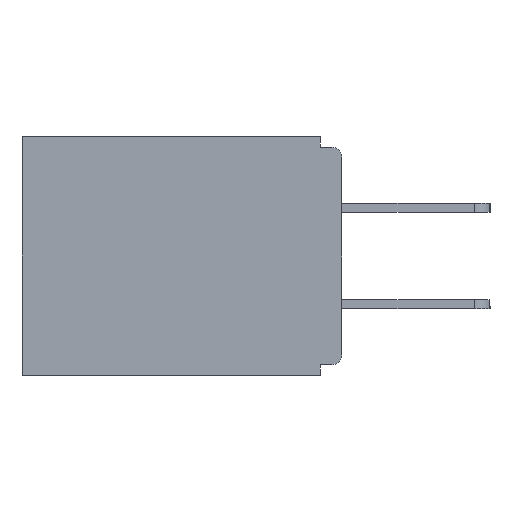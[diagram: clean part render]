
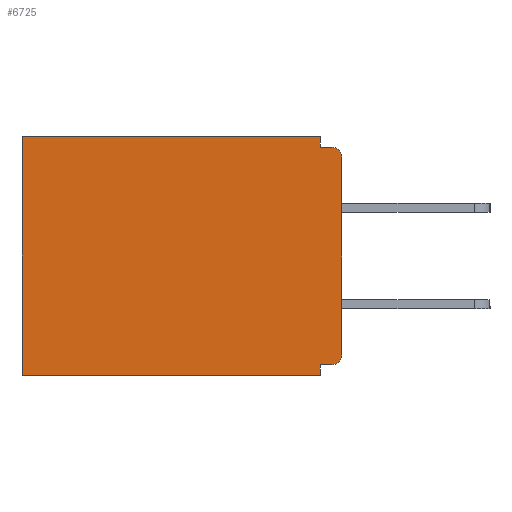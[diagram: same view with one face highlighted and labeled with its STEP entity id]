
A CAD part, left-side view. The second image highlights one B-rep face of the part: STEP entity #6725.
In plain terms, the highlighted planar face has unit normal (-1, 0, 0).
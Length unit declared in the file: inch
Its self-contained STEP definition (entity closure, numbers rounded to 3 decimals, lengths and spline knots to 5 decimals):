
#61 = CARTESIAN_POINT ( 'NONE',  ( 0.298, 0.015, -0.328 ) ) ;
#503 = VERTEX_POINT ( 'NONE', #61 ) ;
#517 = DIRECTION ( 'NONE',  ( 0., 1., 0. ) ) ;
#707 = VECTOR ( 'NONE', #517, 39.37008 ) ;
#1121 = DIRECTION ( 'NONE',  ( -1., 0., 0. ) ) ;
#1235 = AXIS2_PLACEMENT_3D ( 'NONE', #15444, #15633, #13541 ) ;
#2090 = VERTEX_POINT ( 'NONE', #24667 ) ;
#2184 = EDGE_CURVE ( 'NONE', #11422, #6461, #11250, .T. ) ;
#2743 = ORIENTED_EDGE ( 'NONE', *, *, #18848, .F. ) ;
#3019 = ORIENTED_EDGE ( 'NONE', *, *, #14815, .F. ) ;
#3341 = EDGE_CURVE ( 'NONE', #503, #3554, #10534, .T. ) ;
#3554 = VERTEX_POINT ( 'NONE', #15987 ) ;
#3602 = CARTESIAN_POINT ( 'NONE',  ( 0.298, 0.031, -0.343 ) ) ;
#3847 = ORIENTED_EDGE ( 'NONE', *, *, #4492, .F. ) ;
#4006 = CARTESIAN_POINT ( 'NONE',  ( 0.298, 0.015, -0.015 ) ) ;
#4492 = EDGE_CURVE ( 'NONE', #11422, #3554, #22615, .T. ) ;
#4788 = CARTESIAN_POINT ( 'NONE',  ( 0.298, 0., 0. ) ) ;
#5013 = VECTOR ( 'NONE', #8627, 39.37008 ) ;
#5342 = FACE_OUTER_BOUND ( 'NONE', #15247, .T. ) ;
#5429 = DIRECTION ( 'NONE',  ( 0., 1., 0. ) ) ;
#5515 = VERTEX_POINT ( 'NONE', #15365 ) ;
#5703 = EDGE_CURVE ( 'NONE', #17029, #7358, #20069, .T. ) ;
#5813 = ORIENTED_EDGE ( 'NONE', *, *, #6820, .F. ) ;
#6461 = VERTEX_POINT ( 'NONE', #4006 ) ;
#6725 = ADVANCED_FACE ( 'NONE', ( #5342 ), #16725, .F. ) ;
#6820 = EDGE_CURVE ( 'NONE', #2090, #6461, #24026, .T. ) ;
#7358 = VERTEX_POINT ( 'NONE', #18731 ) ;
#7524 = DIRECTION ( 'NONE',  ( 0., 0., -1. ) ) ;
#8010 = AXIS2_PLACEMENT_3D ( 'NONE', #4788, #8545, #16563 ) ;
#8173 = LINE ( 'NONE', #16007, #15008 ) ;
#8213 = ORIENTED_EDGE ( 'NONE', *, *, #20113, .T. ) ;
#8456 = ORIENTED_EDGE ( 'NONE', *, *, #21881, .F. ) ;
#8540 = ORIENTED_EDGE ( 'NONE', *, *, #2184, .T. ) ;
#8545 = DIRECTION ( 'NONE',  ( 1., 0., 0. ) ) ;
#8627 = DIRECTION ( 'NONE',  ( 0., -1., 0. ) ) ;
#8683 = EDGE_CURVE ( 'NONE', #503, #9806, #25272, .T. ) ;
#9072 = DIRECTION ( 'NONE',  ( 0., 0., -1. ) ) ;
#9448 = DIRECTION ( 'NONE',  ( 0., 0., -1. ) ) ;
#9806 = VERTEX_POINT ( 'NONE', #22712 ) ;
#9815 = ORIENTED_EDGE ( 'NONE', *, *, #5703, .T. ) ;
#10089 = DIRECTION ( 'NONE',  ( 0., 0., -1. ) ) ;
#10125 = VECTOR ( 'NONE', #5429, 39.37008 ) ;
#10534 = CIRCLE ( 'NONE', #1235, 0.015 ) ;
#11250 = CIRCLE ( 'NONE', #18789, 0.015 ) ;
#11393 = CARTESIAN_POINT ( 'NONE',  ( 0.298, 0., -0.343 ) ) ;
#11422 = VERTEX_POINT ( 'NONE', #11883 ) ;
#11802 = VECTOR ( 'NONE', #7524, 39.37008 ) ;
#11831 = CARTESIAN_POINT ( 'NONE',  ( 0.298, 0.46, 0. ) ) ;
#11869 = ORIENTED_EDGE ( 'NONE', *, *, #3341, .T. ) ;
#11883 = CARTESIAN_POINT ( 'NONE',  ( 0.298, 0., -0.03 ) ) ;
#13541 = DIRECTION ( 'NONE',  ( 0., 0., -1. ) ) ;
#14635 = CARTESIAN_POINT ( 'NONE',  ( 0.298, 0.031, 0. ) ) ;
#14750 = CARTESIAN_POINT ( 'NONE',  ( 0.298, 0., -0.015 ) ) ;
#14815 = EDGE_CURVE ( 'NONE', #17029, #2090, #22665, .T. ) ;
#15008 = VECTOR ( 'NONE', #19766, 39.37008 ) ;
#15247 = EDGE_LOOP ( 'NONE', ( #8540, #5813, #3019, #9815, #8213, #8456, #2743, #16045, #11869, #3847 ) ) ;
#15365 = CARTESIAN_POINT ( 'NONE',  ( 0.298, 0.031, -0.343 ) ) ;
#15444 = CARTESIAN_POINT ( 'NONE',  ( 0.298, 0.015, -0.313 ) ) ;
#15633 = DIRECTION ( 'NONE',  ( -1., 0., 0. ) ) ;
#15987 = CARTESIAN_POINT ( 'NONE',  ( 0.298, 0., -0.313 ) ) ;
#16007 = CARTESIAN_POINT ( 'NONE',  ( 0.298, 0.031, -0.343 ) ) ;
#16029 = LINE ( 'NONE', #11393, #10125 ) ;
#16045 = ORIENTED_EDGE ( 'NONE', *, *, #8683, .F. ) ;
#16563 = DIRECTION ( 'NONE',  ( 0., 0., -1. ) ) ;
#16725 = PLANE ( 'NONE',  #8010 ) ;
#17029 = VERTEX_POINT ( 'NONE', #14635 ) ;
#17101 = CARTESIAN_POINT ( 'NONE',  ( 0.298, 0.46, -0.343 ) ) ;
#17947 = VERTEX_POINT ( 'NONE', #17101 ) ;
#18412 = CARTESIAN_POINT ( 'NONE',  ( 0.298, 0., 0. ) ) ;
#18460 = CARTESIAN_POINT ( 'NONE',  ( 0.298, 0., -0.328 ) ) ;
#18717 = DIRECTION ( 'NONE',  ( 0., 1., 0. ) ) ;
#18731 = CARTESIAN_POINT ( 'NONE',  ( 0.298, 0.46, 0. ) ) ;
#18789 = AXIS2_PLACEMENT_3D ( 'NONE', #21019, #1121, #9072 ) ;
#18848 = EDGE_CURVE ( 'NONE', #9806, #5515, #8173, .T. ) ;
#19700 = VECTOR ( 'NONE', #18717, 39.37008 ) ;
#19766 = DIRECTION ( 'NONE',  ( 0., 0., -1. ) ) ;
#20069 = LINE ( 'NONE', #18412, #707 ) ;
#20113 = EDGE_CURVE ( 'NONE', #7358, #17947, #25225, .T. ) ;
#21019 = CARTESIAN_POINT ( 'NONE',  ( 0.298, 0.015, -0.03 ) ) ;
#21881 = EDGE_CURVE ( 'NONE', #5515, #17947, #16029, .T. ) ;
#22615 = LINE ( 'NONE', #25109, #25416 ) ;
#22665 = LINE ( 'NONE', #3602, #11802 ) ;
#22712 = CARTESIAN_POINT ( 'NONE',  ( 0.298, 0.031, -0.328 ) ) ;
#23033 = VECTOR ( 'NONE', #10089, 39.37008 ) ;
#24026 = LINE ( 'NONE', #14750, #5013 ) ;
#24667 = CARTESIAN_POINT ( 'NONE',  ( 0.298, 0.031, -0.015 ) ) ;
#25109 = CARTESIAN_POINT ( 'NONE',  ( 0.298, 0., 0. ) ) ;
#25225 = LINE ( 'NONE', #11831, #23033 ) ;
#25272 = LINE ( 'NONE', #18460, #19700 ) ;
#25416 = VECTOR ( 'NONE', #9448, 39.37008 ) ;
